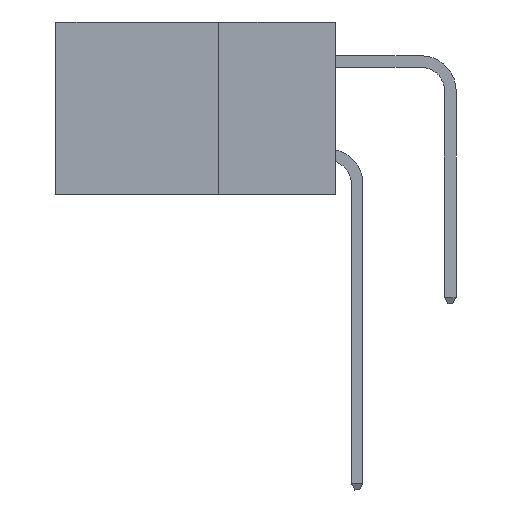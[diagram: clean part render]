
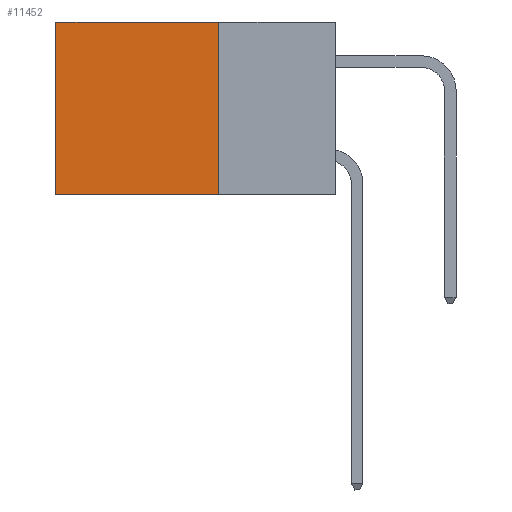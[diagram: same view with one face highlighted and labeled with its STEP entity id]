
A CAD part, left-side view. The second image highlights one B-rep face of the part: STEP entity #11452.
In plain terms, the highlighted planar face has unit normal (-1, 0, 0).
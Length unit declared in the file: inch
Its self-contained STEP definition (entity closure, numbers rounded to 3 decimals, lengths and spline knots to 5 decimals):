
#47 = ORIENTED_EDGE ( 'NONE', *, *, #6676, .T. ) ;
#176 = DIRECTION ( 'NONE',  ( 1., 0., 0. ) ) ;
#569 = DIRECTION ( 'NONE',  ( 0., 1., 0. ) ) ;
#599 = CARTESIAN_POINT ( 'NONE',  ( 0.2875, 0.6, 0. ) ) ;
#862 = VERTEX_POINT ( 'NONE', #19381 ) ;
#1120 = EDGE_LOOP ( 'NONE', ( #5793, #7757, #6573, #47 ) ) ;
#1299 = CARTESIAN_POINT ( 'NONE',  ( 0.2875, 0.25, -0.37 ) ) ;
#1617 = VERTEX_POINT ( 'NONE', #1299 ) ;
#1869 = VECTOR ( 'NONE', #10582, 39.37008 ) ;
#2184 = FACE_OUTER_BOUND ( 'NONE', #1120, .T. ) ;
#3906 = LINE ( 'NONE', #13949, #1869 ) ;
#3923 = VECTOR ( 'NONE', #12809, 39.37008 ) ;
#4052 = DIRECTION ( 'NONE',  ( 0., 0., -1. ) ) ;
#4576 = CARTESIAN_POINT ( 'NONE',  ( 0.2875, 0.25, 0. ) ) ;
#5385 = CARTESIAN_POINT ( 'NONE',  ( 0.2875, 0.25, -0.37 ) ) ;
#5793 = ORIENTED_EDGE ( 'NONE', *, *, #14161, .T. ) ;
#5911 = VERTEX_POINT ( 'NONE', #21072 ) ;
#6573 = ORIENTED_EDGE ( 'NONE', *, *, #12400, .F. ) ;
#6676 = EDGE_CURVE ( 'NONE', #862, #5911, #3906, .T. ) ;
#7438 = VECTOR ( 'NONE', #4052, 39.37008 ) ;
#7757 = ORIENTED_EDGE ( 'NONE', *, *, #10733, .F. ) ;
#7963 = CARTESIAN_POINT ( 'NONE',  ( 0.2875, 0.25, 0. ) ) ;
#8270 = LINE ( 'NONE', #4576, #3923 ) ;
#9552 = CARTESIAN_POINT ( 'NONE',  ( 0.2875, 0.6, -0.37 ) ) ;
#10582 = DIRECTION ( 'NONE',  ( 0., 1., 0. ) ) ;
#10733 = EDGE_CURVE ( 'NONE', #1617, #15420, #21558, .T. ) ;
#11452 = ADVANCED_FACE ( 'NONE', ( #2184 ), #14782, .F. ) ;
#11978 = AXIS2_PLACEMENT_3D ( 'NONE', #7963, #176, #18369 ) ;
#12400 = EDGE_CURVE ( 'NONE', #862, #1617, #8270, .T. ) ;
#12809 = DIRECTION ( 'NONE',  ( 0., 0., -1. ) ) ;
#13949 = CARTESIAN_POINT ( 'NONE',  ( 0.2875, 0.25, 0. ) ) ;
#14161 = EDGE_CURVE ( 'NONE', #5911, #15420, #20047, .T. ) ;
#14782 = PLANE ( 'NONE',  #11978 ) ;
#15420 = VERTEX_POINT ( 'NONE', #9552 ) ;
#16567 = VECTOR ( 'NONE', #569, 39.37008 ) ;
#18369 = DIRECTION ( 'NONE',  ( 0., 0., -1. ) ) ;
#19381 = CARTESIAN_POINT ( 'NONE',  ( 0.2875, 0.25, 0. ) ) ;
#20047 = LINE ( 'NONE', #599, #7438 ) ;
#21072 = CARTESIAN_POINT ( 'NONE',  ( 0.2875, 0.6, 0. ) ) ;
#21558 = LINE ( 'NONE', #5385, #16567 ) ;
